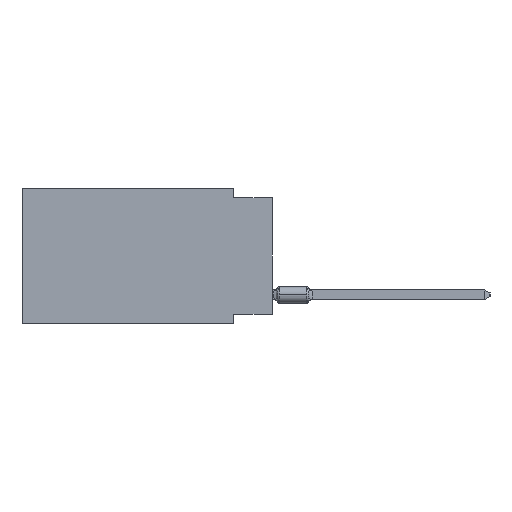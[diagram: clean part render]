
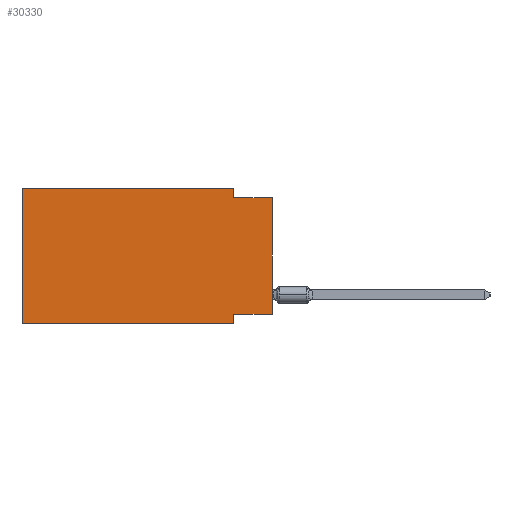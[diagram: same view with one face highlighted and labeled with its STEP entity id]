
A CAD part, left-side view. The second image highlights one B-rep face of the part: STEP entity #30330.
In plain terms, the highlighted planar face has unit normal (-1, 0, 0).
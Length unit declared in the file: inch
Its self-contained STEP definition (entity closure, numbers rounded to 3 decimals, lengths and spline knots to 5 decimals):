
#1382 = CARTESIAN_POINT ( 'NONE',  ( 0., 0., -0.025 ) ) ;
#1402 = CARTESIAN_POINT ( 'NONE',  ( 0., 0., -0.325 ) ) ;
#1465 = ORIENTED_EDGE ( 'NONE', *, *, #16104, .T. ) ;
#2322 = CARTESIAN_POINT ( 'NONE',  ( 0., 0.645, -0.35 ) ) ;
#2656 = CARTESIAN_POINT ( 'NONE',  ( 0., 0.1, 0. ) ) ;
#3766 = LINE ( 'NONE', #1382, #22540 ) ;
#3783 = ORIENTED_EDGE ( 'NONE', *, *, #11586, .F. ) ;
#4611 = EDGE_CURVE ( 'NONE', #7981, #15384, #8153, .T. ) ;
#5237 = VECTOR ( 'NONE', #33741, 39.37008 ) ;
#5533 = CARTESIAN_POINT ( 'NONE',  ( 0., 0.645, 0. ) ) ;
#5551 = VECTOR ( 'NONE', #35595, 39.37008 ) ;
#5998 = VERTEX_POINT ( 'NONE', #42649 ) ;
#6690 = EDGE_CURVE ( 'NONE', #5998, #30967, #3766, .T. ) ;
#7981 = VERTEX_POINT ( 'NONE', #2322 ) ;
#8153 = LINE ( 'NONE', #31641, #5551 ) ;
#8678 = DIRECTION ( 'NONE',  ( 0., 0., -1. ) ) ;
#9032 = CARTESIAN_POINT ( 'NONE',  ( 0., 0.1, -0.325 ) ) ;
#9483 = LINE ( 'NONE', #5533, #5237 ) ;
#10690 = LINE ( 'NONE', #23567, #49814 ) ;
#11432 = EDGE_CURVE ( 'NONE', #16389, #30967, #19404, .T. ) ;
#11586 = EDGE_CURVE ( 'NONE', #41296, #5998, #38529, .T. ) ;
#12632 = LINE ( 'NONE', #36636, #42892 ) ;
#13067 = EDGE_CURVE ( 'NONE', #43796, #26680, #12632, .T. ) ;
#13070 = CARTESIAN_POINT ( 'NONE',  ( 0., 0.1, 0. ) ) ;
#14688 = CARTESIAN_POINT ( 'NONE',  ( 0., 0., 0. ) ) ;
#15384 = VERTEX_POINT ( 'NONE', #23494 ) ;
#16104 = EDGE_CURVE ( 'NONE', #7981, #26680, #10690, .T. ) ;
#16389 = VERTEX_POINT ( 'NONE', #1402 ) ;
#16707 = DIRECTION ( 'NONE',  ( 1., 0., 0. ) ) ;
#17752 = ORIENTED_EDGE ( 'NONE', *, *, #11432, .T. ) ;
#18666 = EDGE_LOOP ( 'NONE', ( #17752, #38600, #3783, #37289, #38230, #1465, #47092, #27445 ) ) ;
#19404 = LINE ( 'NONE', #14688, #36997 ) ;
#21291 = VECTOR ( 'NONE', #46675, 39.37008 ) ;
#22540 = VECTOR ( 'NONE', #29850, 39.37008 ) ;
#23494 = CARTESIAN_POINT ( 'NONE',  ( 0., 0.645, 0. ) ) ;
#23567 = CARTESIAN_POINT ( 'NONE',  ( 0., 0.645, -0.35 ) ) ;
#24340 = VECTOR ( 'NONE', #34834, 39.37008 ) ;
#26680 = VERTEX_POINT ( 'NONE', #52012 ) ;
#27445 = ORIENTED_EDGE ( 'NONE', *, *, #37736, .F. ) ;
#27554 = DIRECTION ( 'NONE',  ( 0., -1., 0. ) ) ;
#29850 = DIRECTION ( 'NONE',  ( 0., -1., 0. ) ) ;
#30330 = ADVANCED_FACE ( 'NONE', ( #36765 ), #44923, .F. ) ;
#30599 = CARTESIAN_POINT ( 'NONE',  ( 0., 0., -0.325 ) ) ;
#30765 = DIRECTION ( 'NONE',  ( 0., 0., 1. ) ) ;
#30967 = VERTEX_POINT ( 'NONE', #38292 ) ;
#31416 = EDGE_CURVE ( 'NONE', #15384, #41296, #9483, .T. ) ;
#31641 = CARTESIAN_POINT ( 'NONE',  ( 0., 0.645, 0. ) ) ;
#32030 = DIRECTION ( 'NONE',  ( 0., 0., -1. ) ) ;
#33741 = DIRECTION ( 'NONE',  ( 0., -1., 0. ) ) ;
#34834 = DIRECTION ( 'NONE',  ( 0., 0., -1. ) ) ;
#35595 = DIRECTION ( 'NONE',  ( 0., 0., 1. ) ) ;
#36636 = CARTESIAN_POINT ( 'NONE',  ( 0., 0.1, -0.35 ) ) ;
#36765 = FACE_OUTER_BOUND ( 'NONE', #18666, .T. ) ;
#36997 = VECTOR ( 'NONE', #30765, 39.37008 ) ;
#37289 = ORIENTED_EDGE ( 'NONE', *, *, #31416, .F. ) ;
#37736 = EDGE_CURVE ( 'NONE', #16389, #43796, #50633, .T. ) ;
#38230 = ORIENTED_EDGE ( 'NONE', *, *, #4611, .F. ) ;
#38292 = CARTESIAN_POINT ( 'NONE',  ( 0., 0., -0.025 ) ) ;
#38529 = LINE ( 'NONE', #2656, #24340 ) ;
#38600 = ORIENTED_EDGE ( 'NONE', *, *, #6690, .F. ) ;
#40623 = AXIS2_PLACEMENT_3D ( 'NONE', #45187, #16707, #32030 ) ;
#41296 = VERTEX_POINT ( 'NONE', #13070 ) ;
#42649 = CARTESIAN_POINT ( 'NONE',  ( 0., 0.1, -0.025 ) ) ;
#42892 = VECTOR ( 'NONE', #8678, 39.37008 ) ;
#43796 = VERTEX_POINT ( 'NONE', #9032 ) ;
#44923 = PLANE ( 'NONE',  #40623 ) ;
#45187 = CARTESIAN_POINT ( 'NONE',  ( 0., 0.645, 0. ) ) ;
#46675 = DIRECTION ( 'NONE',  ( 0., 1., 0. ) ) ;
#47092 = ORIENTED_EDGE ( 'NONE', *, *, #13067, .F. ) ;
#49814 = VECTOR ( 'NONE', #27554, 39.37008 ) ;
#50633 = LINE ( 'NONE', #30599, #21291 ) ;
#52012 = CARTESIAN_POINT ( 'NONE',  ( 0., 0.1, -0.35 ) ) ;
